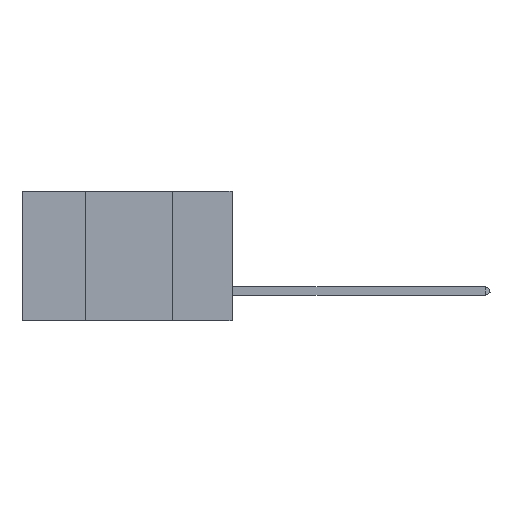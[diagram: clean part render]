
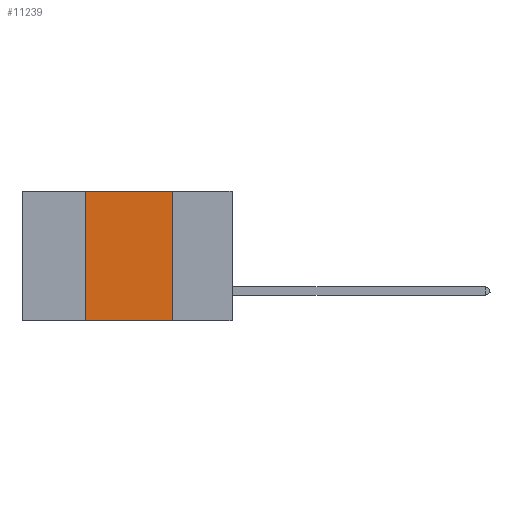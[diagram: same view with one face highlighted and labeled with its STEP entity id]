
A CAD part, left-side view. The second image highlights one B-rep face of the part: STEP entity #11239.
In plain terms, the highlighted planar face has unit normal (-1, 0, 0).
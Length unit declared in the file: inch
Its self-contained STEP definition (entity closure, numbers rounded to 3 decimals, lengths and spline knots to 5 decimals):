
#919 = VERTEX_POINT ( 'NONE', #3968 ) ;
#1538 = ORIENTED_EDGE ( 'NONE', *, *, #21317, .F. ) ;
#2096 = VECTOR ( 'NONE', #22057, 39.37008 ) ;
#2634 = DIRECTION ( 'NONE',  ( 0., 0., -1. ) ) ;
#2639 = ORIENTED_EDGE ( 'NONE', *, *, #8654, .T. ) ;
#3968 = CARTESIAN_POINT ( 'NONE',  ( 0., 0.42, -0.37 ) ) ;
#3984 = VERTEX_POINT ( 'NONE', #5370 ) ;
#4645 = CARTESIAN_POINT ( 'NONE',  ( 0., 0.6, 0. ) ) ;
#5370 = CARTESIAN_POINT ( 'NONE',  ( 0., 0.42, 0. ) ) ;
#5879 = CARTESIAN_POINT ( 'NONE',  ( 0., 0.6, -0.37 ) ) ;
#6096 = VECTOR ( 'NONE', #20441, 39.37008 ) ;
#6383 = LINE ( 'NONE', #12807, #2096 ) ;
#6568 = VECTOR ( 'NONE', #10751, 39.37008 ) ;
#8308 = CARTESIAN_POINT ( 'NONE',  ( 0., 0.17, -0.37 ) ) ;
#8654 = EDGE_CURVE ( 'NONE', #919, #10805, #10994, .T. ) ;
#9132 = VECTOR ( 'NONE', #16851, 39.37008 ) ;
#9718 = VERTEX_POINT ( 'NONE', #11711 ) ;
#10751 = DIRECTION ( 'NONE',  ( 0., -1., 0. ) ) ;
#10805 = VERTEX_POINT ( 'NONE', #8308 ) ;
#10994 = LINE ( 'NONE', #5879, #6096 ) ;
#11239 = ADVANCED_FACE ( 'NONE', ( #12003 ), #14414, .F. ) ;
#11504 = EDGE_LOOP ( 'NONE', ( #20459, #19259, #1538, #2639 ) ) ;
#11711 = CARTESIAN_POINT ( 'NONE',  ( 0., 0.17, 0. ) ) ;
#12003 = FACE_OUTER_BOUND ( 'NONE', #11504, .T. ) ;
#12025 = LINE ( 'NONE', #13484, #6568 ) ;
#12807 = CARTESIAN_POINT ( 'NONE',  ( 0., 0.42, 0. ) ) ;
#13484 = CARTESIAN_POINT ( 'NONE',  ( 0., 0.6, 0. ) ) ;
#13748 = DIRECTION ( 'NONE',  ( 1., 0., 0. ) ) ;
#13933 = LINE ( 'NONE', #18914, #9132 ) ;
#14414 = PLANE ( 'NONE',  #16787 ) ;
#16731 = EDGE_CURVE ( 'NONE', #3984, #9718, #12025, .T. ) ;
#16787 = AXIS2_PLACEMENT_3D ( 'NONE', #4645, #13748, #2634 ) ;
#16851 = DIRECTION ( 'NONE',  ( 0., 0., -1. ) ) ;
#18592 = EDGE_CURVE ( 'NONE', #9718, #10805, #13933, .T. ) ;
#18914 = CARTESIAN_POINT ( 'NONE',  ( 0., 0.17, 0. ) ) ;
#19259 = ORIENTED_EDGE ( 'NONE', *, *, #16731, .F. ) ;
#20441 = DIRECTION ( 'NONE',  ( 0., -1., 0. ) ) ;
#20459 = ORIENTED_EDGE ( 'NONE', *, *, #18592, .F. ) ;
#21317 = EDGE_CURVE ( 'NONE', #919, #3984, #6383, .T. ) ;
#22057 = DIRECTION ( 'NONE',  ( 0., 0., 1. ) ) ;
